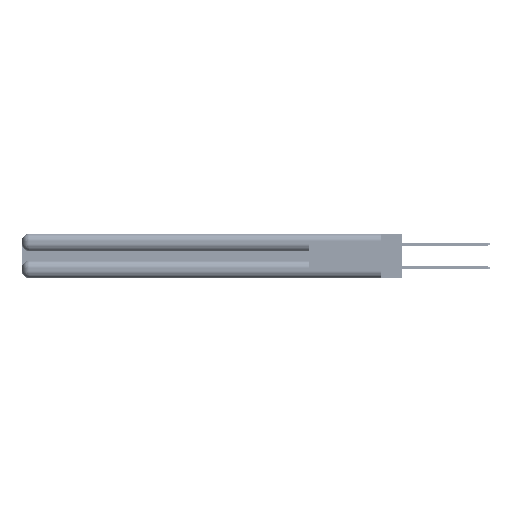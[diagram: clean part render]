
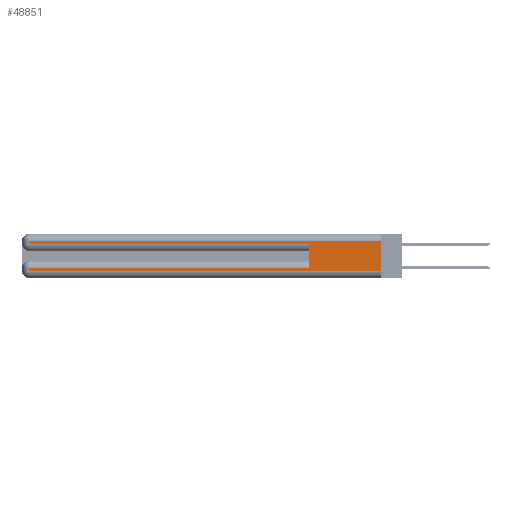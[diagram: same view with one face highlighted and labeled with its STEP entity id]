
A CAD part, left-side view. The second image highlights one B-rep face of the part: STEP entity #48851.
In plain terms, the highlighted planar face has unit normal (-1, 0, 0).
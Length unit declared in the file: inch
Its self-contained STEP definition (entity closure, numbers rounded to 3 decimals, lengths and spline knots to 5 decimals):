
#636 = DIRECTION ( 'NONE',  ( 1., 0., 0. ) ) ;
#759 = LINE ( 'NONE', #20768, #46342 ) ;
#1233 = CARTESIAN_POINT ( 'NONE',  ( 0., 0., 0.285 ) ) ;
#1499 = EDGE_CURVE ( 'NONE', #31777, #44733, #16845, .T. ) ;
#2786 = AXIS2_PLACEMENT_3D ( 'NONE', #27111, #636, #31568 ) ;
#2939 = CARTESIAN_POINT ( 'NONE',  ( 0., 2.94, 0.06 ) ) ;
#5456 = VERTEX_POINT ( 'NONE', #2939 ) ;
#6032 = DIRECTION ( 'NONE',  ( 0., -1., 0. ) ) ;
#6786 = CARTESIAN_POINT ( 'NONE',  ( 0., 0., 0.31 ) ) ;
#8577 = ORIENTED_EDGE ( 'NONE', *, *, #51851, .T. ) ;
#8827 = LINE ( 'NONE', #17948, #28222 ) ;
#9910 = VECTOR ( 'NONE', #19299, 39.37008 ) ;
#11469 = CARTESIAN_POINT ( 'NONE',  ( 0., 2.94, 0.085 ) ) ;
#12383 = CARTESIAN_POINT ( 'NONE',  ( 0., 0.6, 0.085 ) ) ;
#15089 = EDGE_LOOP ( 'NONE', ( #37337, #22596, #15599, #40910, #20148, #24189, #45158, #8577 ) ) ;
#15599 = ORIENTED_EDGE ( 'NONE', *, *, #28315, .T. ) ;
#15614 = DIRECTION ( 'NONE',  ( 0., 1., 0. ) ) ;
#16845 = LINE ( 'NONE', #1233, #45180 ) ;
#17150 = LINE ( 'NONE', #54541, #41974 ) ;
#17948 = CARTESIAN_POINT ( 'NONE',  ( 0., 0., 0.37 ) ) ;
#18174 = PLANE ( 'NONE',  #2786 ) ;
#18880 = EDGE_CURVE ( 'NONE', #47112, #31611, #46733, .T. ) ;
#19299 = DIRECTION ( 'NONE',  ( 0., -1., 0. ) ) ;
#19310 = CARTESIAN_POINT ( 'NONE',  ( 0., 0.6, 0.145 ) ) ;
#20148 = ORIENTED_EDGE ( 'NONE', *, *, #34572, .F. ) ;
#20768 = CARTESIAN_POINT ( 'NONE',  ( 0., 2.94, 0.37 ) ) ;
#20800 = CARTESIAN_POINT ( 'NONE',  ( 0., 0., 0.31 ) ) ;
#22596 = ORIENTED_EDGE ( 'NONE', *, *, #18880, .T. ) ;
#22808 = DIRECTION ( 'NONE',  ( 0., 0., -1. ) ) ;
#23089 = LINE ( 'NONE', #41681, #9910 ) ;
#24189 = ORIENTED_EDGE ( 'NONE', *, *, #37972, .T. ) ;
#25608 = CARTESIAN_POINT ( 'NONE',  ( 0., 0.6, 0.285 ) ) ;
#27111 = CARTESIAN_POINT ( 'NONE',  ( 0., 0., 0.37 ) ) ;
#27462 = DIRECTION ( 'NONE',  ( 0., 0., 1. ) ) ;
#27540 = VERTEX_POINT ( 'NONE', #49996 ) ;
#28222 = VECTOR ( 'NONE', #22808, 39.37008 ) ;
#28315 = EDGE_CURVE ( 'NONE', #31611, #31777, #17150, .T. ) ;
#29187 = VERTEX_POINT ( 'NONE', #12383 ) ;
#31568 = DIRECTION ( 'NONE',  ( 0., 0., -1. ) ) ;
#31611 = VERTEX_POINT ( 'NONE', #47123 ) ;
#31777 = VERTEX_POINT ( 'NONE', #57128 ) ;
#32034 = FACE_OUTER_BOUND ( 'NONE', #15089, .T. ) ;
#34572 = EDGE_CURVE ( 'NONE', #29187, #44733, #51025, .T. ) ;
#36534 = VECTOR ( 'NONE', #27462, 39.37008 ) ;
#37337 = ORIENTED_EDGE ( 'NONE', *, *, #45618, .F. ) ;
#37972 = EDGE_CURVE ( 'NONE', #29187, #40181, #45905, .T. ) ;
#40181 = VERTEX_POINT ( 'NONE', #11469 ) ;
#40910 = ORIENTED_EDGE ( 'NONE', *, *, #1499, .T. ) ;
#41162 = VECTOR ( 'NONE', #46689, 39.37008 ) ;
#41420 = DIRECTION ( 'NONE',  ( 0., 0., -1. ) ) ;
#41681 = CARTESIAN_POINT ( 'NONE',  ( 0., 0., 0.06 ) ) ;
#41974 = VECTOR ( 'NONE', #41420, 39.37008 ) ;
#44733 = VERTEX_POINT ( 'NONE', #25608 ) ;
#45158 = ORIENTED_EDGE ( 'NONE', *, *, #54215, .T. ) ;
#45180 = VECTOR ( 'NONE', #6032, 39.37008 ) ;
#45618 = EDGE_CURVE ( 'NONE', #47112, #27540, #8827, .T. ) ;
#45905 = LINE ( 'NONE', #51508, #55568 ) ;
#46342 = VECTOR ( 'NONE', #52377, 39.37008 ) ;
#46689 = DIRECTION ( 'NONE',  ( 0., 1., 0. ) ) ;
#46733 = LINE ( 'NONE', #20800, #41162 ) ;
#47112 = VERTEX_POINT ( 'NONE', #6786 ) ;
#47123 = CARTESIAN_POINT ( 'NONE',  ( 0., 2.94, 0.31 ) ) ;
#48851 = ADVANCED_FACE ( 'NONE', ( #32034 ), #18174, .F. ) ;
#49996 = CARTESIAN_POINT ( 'NONE',  ( 0., 0., 0.06 ) ) ;
#51025 = LINE ( 'NONE', #19310, #36534 ) ;
#51508 = CARTESIAN_POINT ( 'NONE',  ( 0., 0., 0.085 ) ) ;
#51851 = EDGE_CURVE ( 'NONE', #5456, #27540, #23089, .T. ) ;
#52377 = DIRECTION ( 'NONE',  ( 0., 0., -1. ) ) ;
#54215 = EDGE_CURVE ( 'NONE', #40181, #5456, #759, .T. ) ;
#54541 = CARTESIAN_POINT ( 'NONE',  ( 0., 2.94, 0.37 ) ) ;
#55568 = VECTOR ( 'NONE', #15614, 39.37008 ) ;
#57128 = CARTESIAN_POINT ( 'NONE',  ( 0., 2.94, 0.285 ) ) ;
